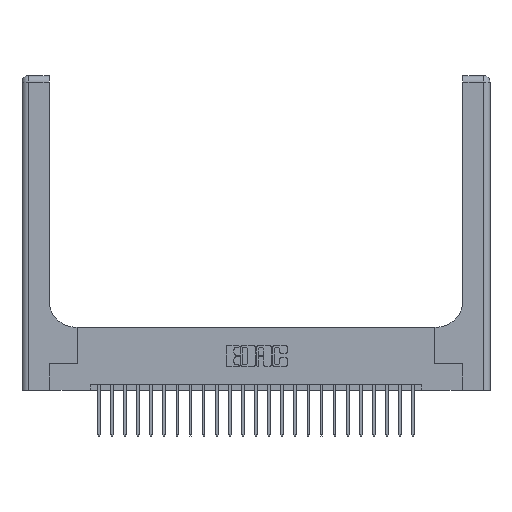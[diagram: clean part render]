
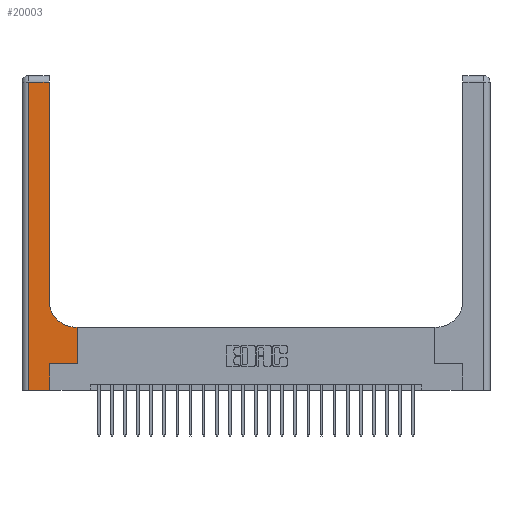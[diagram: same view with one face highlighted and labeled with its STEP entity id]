
A CAD part, top view. The second image highlights one B-rep face of the part: STEP entity #20003.
In plain terms, the highlighted planar face has unit normal (0, 0, 1).
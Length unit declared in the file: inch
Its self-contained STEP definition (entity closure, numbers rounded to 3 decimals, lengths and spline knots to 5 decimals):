
#7 = VERTEX_POINT ( 'NONE', #4519 ) ;
#132 = CARTESIAN_POINT ( 'NONE',  ( 0.06, 3., 0.37 ) ) ;
#383 = DIRECTION ( 'NONE',  ( 0., 0., -1. ) ) ;
#752 = LINE ( 'NONE', #6389, #24039 ) ;
#981 = DIRECTION ( 'NONE',  ( -1., 0., 0. ) ) ;
#1021 = CARTESIAN_POINT ( 'NONE',  ( 0.26, 0.85, 0.37 ) ) ;
#1405 = VECTOR ( 'NONE', #7200, 39.37008 ) ;
#2581 = LINE ( 'NONE', #17820, #21877 ) ;
#2812 = LINE ( 'NONE', #8462, #18561 ) ;
#3238 = VERTEX_POINT ( 'NONE', #1021 ) ;
#3587 = EDGE_CURVE ( 'NONE', #18076, #6238, #21031, .T. ) ;
#3935 = DIRECTION ( 'NONE',  ( 0., 1., 0. ) ) ;
#4519 = CARTESIAN_POINT ( 'NONE',  ( 0.265, 0.25, 0.37 ) ) ;
#4567 = VERTEX_POINT ( 'NONE', #9107 ) ;
#4830 = EDGE_CURVE ( 'NONE', #4567, #16561, #2581, .T. ) ;
#4898 = CARTESIAN_POINT ( 'NONE',  ( 0.26, 3., 0.37 ) ) ;
#5422 = LINE ( 'NONE', #20547, #20241 ) ;
#5517 = LINE ( 'NONE', #132, #22987 ) ;
#5648 = DIRECTION ( 'NONE',  ( 1., 0., 0. ) ) ;
#5740 = ORIENTED_EDGE ( 'NONE', *, *, #10124, .T. ) ;
#6007 = CARTESIAN_POINT ( 'NONE',  ( 0.51, 0.85, 0.37 ) ) ;
#6238 = VERTEX_POINT ( 'NONE', #8848 ) ;
#6307 = DIRECTION ( 'NONE',  ( 0., 0., -1. ) ) ;
#6389 = CARTESIAN_POINT ( 'NONE',  ( 0.265, 0.25, 0.37 ) ) ;
#6640 = LINE ( 'NONE', #15751, #7244 ) ;
#7200 = DIRECTION ( 'NONE',  ( 0., 1., 0. ) ) ;
#7244 = VECTOR ( 'NONE', #11942, 39.37008 ) ;
#7550 = AXIS2_PLACEMENT_3D ( 'NONE', #6007, #383, #9974 ) ;
#8231 = CARTESIAN_POINT ( 'NONE',  ( 0.06, 0., 0.37 ) ) ;
#8243 = CARTESIAN_POINT ( 'NONE',  ( 0.51, 0.6, 0.37 ) ) ;
#8462 = CARTESIAN_POINT ( 'NONE',  ( 0.26, 0.6, 0.37 ) ) ;
#8629 = EDGE_CURVE ( 'NONE', #6238, #7, #6640, .T. ) ;
#8663 = ORIENTED_EDGE ( 'NONE', *, *, #8629, .T. ) ;
#8848 = CARTESIAN_POINT ( 'NONE',  ( 0.265, 0., 0.37 ) ) ;
#9107 = CARTESIAN_POINT ( 'NONE',  ( 0.26, 2.94, 0.37 ) ) ;
#9186 = DIRECTION ( 'NONE',  ( -1., 0., 0. ) ) ;
#9313 = CARTESIAN_POINT ( 'NONE',  ( 0., 3., 0.37 ) ) ;
#9772 = VERTEX_POINT ( 'NONE', #8243 ) ;
#9974 = DIRECTION ( 'NONE',  ( 1., 0., 0. ) ) ;
#10124 = EDGE_CURVE ( 'NONE', #16561, #18076, #5517, .T. ) ;
#10550 = EDGE_CURVE ( 'NONE', #3238, #4567, #21993, .T. ) ;
#11025 = FACE_OUTER_BOUND ( 'NONE', #19210, .T. ) ;
#11134 = ORIENTED_EDGE ( 'NONE', *, *, #10550, .T. ) ;
#11278 = VERTEX_POINT ( 'NONE', #20289 ) ;
#11420 = DIRECTION ( 'NONE',  ( 0., -1., 0. ) ) ;
#11600 = ORIENTED_EDGE ( 'NONE', *, *, #18209, .T. ) ;
#11852 = PLANE ( 'NONE',  #20231 ) ;
#11923 = DIRECTION ( 'NONE',  ( -1., 0., 0. ) ) ;
#11942 = DIRECTION ( 'NONE',  ( 0., 1., 0. ) ) ;
#13008 = VERTEX_POINT ( 'NONE', #22817 ) ;
#13153 = CARTESIAN_POINT ( 'NONE',  ( 0., 0., 0.37 ) ) ;
#13905 = DIRECTION ( 'NONE',  ( 1., 0., 0. ) ) ;
#14273 = CIRCLE ( 'NONE', #7550, 0.25 ) ;
#14742 = VECTOR ( 'NONE', #5648, 39.37008 ) ;
#15686 = ORIENTED_EDGE ( 'NONE', *, *, #3587, .T. ) ;
#15751 = CARTESIAN_POINT ( 'NONE',  ( 0.265, 0., 0.37 ) ) ;
#16561 = VERTEX_POINT ( 'NONE', #18340 ) ;
#16570 = EDGE_CURVE ( 'NONE', #13008, #11278, #5422, .T. ) ;
#17084 = ORIENTED_EDGE ( 'NONE', *, *, #22011, .T. ) ;
#17820 = CARTESIAN_POINT ( 'NONE',  ( 0., 2.94, 0.37 ) ) ;
#18076 = VERTEX_POINT ( 'NONE', #8231 ) ;
#18209 = EDGE_CURVE ( 'NONE', #7, #13008, #752, .T. ) ;
#18340 = CARTESIAN_POINT ( 'NONE',  ( 0.06, 2.94, 0.37 ) ) ;
#18561 = VECTOR ( 'NONE', #981, 39.37008 ) ;
#19210 = EDGE_LOOP ( 'NONE', ( #11134, #20109, #5740, #15686, #8663, #11600, #23631, #20662, #17084 ) ) ;
#20003 = ADVANCED_FACE ( 'NONE', ( #11025 ), #11852, .F. ) ;
#20109 = ORIENTED_EDGE ( 'NONE', *, *, #4830, .T. ) ;
#20231 = AXIS2_PLACEMENT_3D ( 'NONE', #9313, #6307, #9186 ) ;
#20241 = VECTOR ( 'NONE', #3935, 39.37008 ) ;
#20289 = CARTESIAN_POINT ( 'NONE',  ( 0.528, 0.6, 0.37 ) ) ;
#20547 = CARTESIAN_POINT ( 'NONE',  ( 0.528, 0.25, 0.37 ) ) ;
#20662 = ORIENTED_EDGE ( 'NONE', *, *, #24049, .T. ) ;
#21031 = LINE ( 'NONE', #13153, #14742 ) ;
#21877 = VECTOR ( 'NONE', #11923, 39.37008 ) ;
#21993 = LINE ( 'NONE', #4898, #1405 ) ;
#22011 = EDGE_CURVE ( 'NONE', #9772, #3238, #14273, .T. ) ;
#22817 = CARTESIAN_POINT ( 'NONE',  ( 0.528, 0.25, 0.37 ) ) ;
#22987 = VECTOR ( 'NONE', #11420, 39.37008 ) ;
#23631 = ORIENTED_EDGE ( 'NONE', *, *, #16570, .T. ) ;
#24039 = VECTOR ( 'NONE', #13905, 39.37008 ) ;
#24049 = EDGE_CURVE ( 'NONE', #11278, #9772, #2812, .T. ) ;
